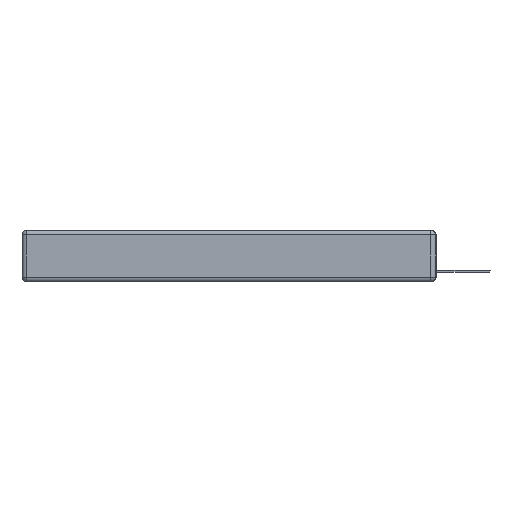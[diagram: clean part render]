
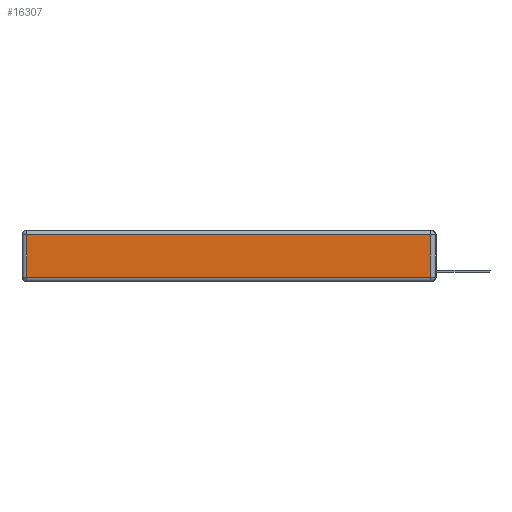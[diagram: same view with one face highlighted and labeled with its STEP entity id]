
A CAD part, left-side view. The second image highlights one B-rep face of the part: STEP entity #16307.
In plain terms, the highlighted planar face has unit normal (-1, 0, 0).
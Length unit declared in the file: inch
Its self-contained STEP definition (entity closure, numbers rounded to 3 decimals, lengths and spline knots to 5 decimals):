
#915 = CARTESIAN_POINT ( 'NONE',  ( 0., 2.72, -0.343 ) ) ;
#924 = PLANE ( 'NONE',  #9967 ) ;
#2246 = CARTESIAN_POINT ( 'NONE',  ( 0., 0., -0.343 ) ) ;
#2863 = VERTEX_POINT ( 'NONE', #6351 ) ;
#3374 = DIRECTION ( 'NONE',  ( 0., 0., -1. ) ) ;
#4108 = CARTESIAN_POINT ( 'NONE',  ( 0., 0.03, -0.343 ) ) ;
#4249 = CARTESIAN_POINT ( 'NONE',  ( 0., 0.03, -0.03 ) ) ;
#4560 = VERTEX_POINT ( 'NONE', #16780 ) ;
#4619 = EDGE_CURVE ( 'NONE', #5198, #7303, #13701, .T. ) ;
#5198 = VERTEX_POINT ( 'NONE', #6141 ) ;
#5537 = ORIENTED_EDGE ( 'NONE', *, *, #9870, .T. ) ;
#5986 = EDGE_CURVE ( 'NONE', #7303, #2863, #9075, .T. ) ;
#6141 = CARTESIAN_POINT ( 'NONE',  ( 0., 0.03, -0.313 ) ) ;
#6351 = CARTESIAN_POINT ( 'NONE',  ( 0., 2.72, -0.03 ) ) ;
#7303 = VERTEX_POINT ( 'NONE', #4249 ) ;
#7530 = DIRECTION ( 'NONE',  ( 0., -1., 0. ) ) ;
#8561 = DIRECTION ( 'NONE',  ( 0., 0., 1. ) ) ;
#9075 = LINE ( 'NONE', #9246, #13380 ) ;
#9246 = CARTESIAN_POINT ( 'NONE',  ( 0., 2.75, -0.03 ) ) ;
#9870 = EDGE_CURVE ( 'NONE', #2863, #4560, #16952, .T. ) ;
#9872 = EDGE_CURVE ( 'NONE', #4560, #5198, #14098, .T. ) ;
#9967 = AXIS2_PLACEMENT_3D ( 'NONE', #2246, #17904, #17777 ) ;
#10534 = DIRECTION ( 'NONE',  ( 0., 1., 0. ) ) ;
#10701 = VECTOR ( 'NONE', #8561, 39.37008 ) ;
#11383 = FACE_OUTER_BOUND ( 'NONE', #13391, .T. ) ;
#12173 = VECTOR ( 'NONE', #7530, 39.37008 ) ;
#13380 = VECTOR ( 'NONE', #10534, 39.37008 ) ;
#13391 = EDGE_LOOP ( 'NONE', ( #16722, #14916, #17035, #5537 ) ) ;
#13701 = LINE ( 'NONE', #4108, #10701 ) ;
#14098 = LINE ( 'NONE', #15945, #12173 ) ;
#14916 = ORIENTED_EDGE ( 'NONE', *, *, #4619, .T. ) ;
#15883 = VECTOR ( 'NONE', #3374, 39.37008 ) ;
#15945 = CARTESIAN_POINT ( 'NONE',  ( 0., 0., -0.313 ) ) ;
#16307 = ADVANCED_FACE ( 'NONE', ( #11383 ), #924, .T. ) ;
#16722 = ORIENTED_EDGE ( 'NONE', *, *, #9872, .T. ) ;
#16780 = CARTESIAN_POINT ( 'NONE',  ( 0., 2.72, -0.313 ) ) ;
#16952 = LINE ( 'NONE', #915, #15883 ) ;
#17035 = ORIENTED_EDGE ( 'NONE', *, *, #5986, .T. ) ;
#17777 = DIRECTION ( 'NONE',  ( 0., 0., 1. ) ) ;
#17904 = DIRECTION ( 'NONE',  ( -1., 0., 0. ) ) ;
